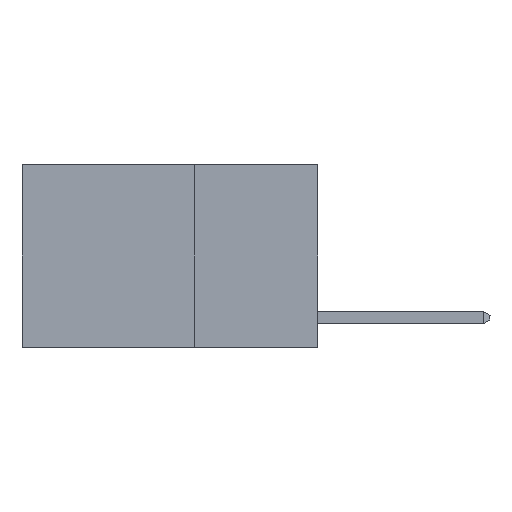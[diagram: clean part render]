
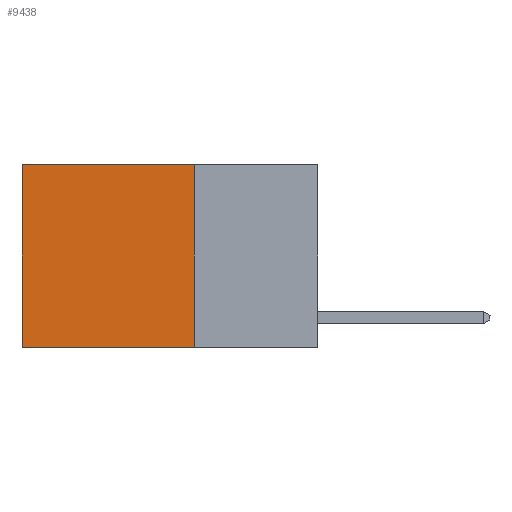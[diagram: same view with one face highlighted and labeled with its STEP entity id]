
A CAD part, left-side view. The second image highlights one B-rep face of the part: STEP entity #9438.
In plain terms, the highlighted planar face has unit normal (-1, 0, 0).
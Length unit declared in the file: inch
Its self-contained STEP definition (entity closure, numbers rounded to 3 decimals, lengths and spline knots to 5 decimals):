
#35 = ORIENTED_EDGE ( 'NONE', *, *, #5837, .T. ) ;
#180 = VERTEX_POINT ( 'NONE', #2037 ) ;
#197 = ORIENTED_EDGE ( 'NONE', *, *, #4323, .T. ) ;
#299 = EDGE_LOOP ( 'NONE', ( #197, #7935, #13389, #35 ) ) ;
#419 = AXIS2_PLACEMENT_3D ( 'NONE', #791, #13324, #4917 ) ;
#791 = CARTESIAN_POINT ( 'NONE',  ( 0.2625, 0.25, 0. ) ) ;
#1925 = DIRECTION ( 'NONE',  ( 0., 0., -1. ) ) ;
#2037 = CARTESIAN_POINT ( 'NONE',  ( 0.2625, 0.6, 0. ) ) ;
#2133 = CARTESIAN_POINT ( 'NONE',  ( 0.2625, 0.6, 0. ) ) ;
#2354 = VECTOR ( 'NONE', #5495, 39.37008 ) ;
#2620 = LINE ( 'NONE', #4429, #10395 ) ;
#3052 = PLANE ( 'NONE',  #419 ) ;
#3990 = EDGE_CURVE ( 'NONE', #4439, #5079, #2620, .T. ) ;
#4307 = DIRECTION ( 'NONE',  ( 0., 1., 0. ) ) ;
#4323 = EDGE_CURVE ( 'NONE', #180, #12944, #11172, .T. ) ;
#4333 = CARTESIAN_POINT ( 'NONE',  ( 0.2625, 0.25, -0.37 ) ) ;
#4419 = LINE ( 'NONE', #12888, #2354 ) ;
#4429 = CARTESIAN_POINT ( 'NONE',  ( 0.2625, 0.25, 0. ) ) ;
#4439 = VERTEX_POINT ( 'NONE', #11703 ) ;
#4917 = DIRECTION ( 'NONE',  ( 0., 0., -1. ) ) ;
#5079 = VERTEX_POINT ( 'NONE', #4333 ) ;
#5495 = DIRECTION ( 'NONE',  ( 0., 1., 0. ) ) ;
#5837 = EDGE_CURVE ( 'NONE', #4439, #180, #12086, .T. ) ;
#5921 = FACE_OUTER_BOUND ( 'NONE', #299, .T. ) ;
#6920 = CARTESIAN_POINT ( 'NONE',  ( 0.2625, 0.25, 0. ) ) ;
#7766 = EDGE_CURVE ( 'NONE', #5079, #12944, #4419, .T. ) ;
#7935 = ORIENTED_EDGE ( 'NONE', *, *, #7766, .F. ) ;
#9192 = CARTESIAN_POINT ( 'NONE',  ( 0.2625, 0.6, -0.37 ) ) ;
#9438 = ADVANCED_FACE ( 'NONE', ( #5921 ), #3052, .F. ) ;
#10395 = VECTOR ( 'NONE', #10574, 39.37008 ) ;
#10574 = DIRECTION ( 'NONE',  ( 0., 0., -1. ) ) ;
#11172 = LINE ( 'NONE', #2133, #12576 ) ;
#11703 = CARTESIAN_POINT ( 'NONE',  ( 0.2625, 0.25, 0. ) ) ;
#12086 = LINE ( 'NONE', #6920, #12234 ) ;
#12234 = VECTOR ( 'NONE', #4307, 39.37008 ) ;
#12576 = VECTOR ( 'NONE', #1925, 39.37008 ) ;
#12888 = CARTESIAN_POINT ( 'NONE',  ( 0.2625, 0.25, -0.37 ) ) ;
#12944 = VERTEX_POINT ( 'NONE', #9192 ) ;
#13324 = DIRECTION ( 'NONE',  ( 1., 0., 0. ) ) ;
#13389 = ORIENTED_EDGE ( 'NONE', *, *, #3990, .F. ) ;
